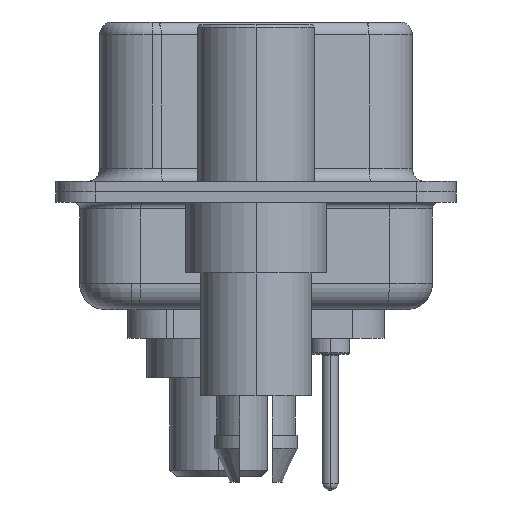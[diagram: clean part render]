
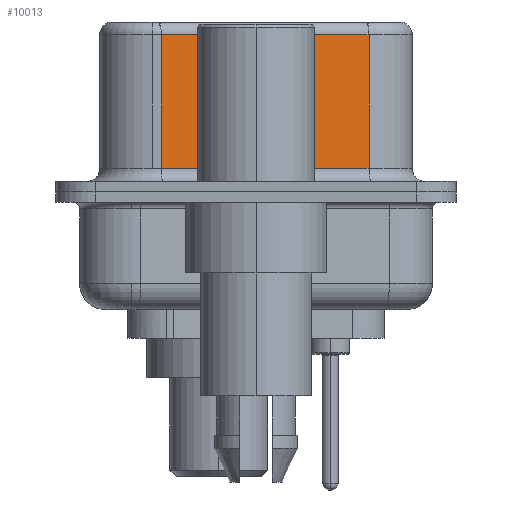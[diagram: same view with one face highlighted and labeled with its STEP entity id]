
A CAD part, left-side view. The second image highlights one B-rep face of the part: STEP entity #10013.
In plain terms, the highlighted planar face has unit normal (-0.985, -0.174, 0).
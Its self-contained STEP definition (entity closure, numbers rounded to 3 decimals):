
#69 = DIRECTION ( 'NONE',  ( 0.174, -0.985, 0. ) ) ;
#241 = VERTEX_POINT ( 'NONE', #258 ) ;
#258 = CARTESIAN_POINT ( 'NONE',  ( 3.73, 3.628, 0.9 ) ) ;
#412 = VERTEX_POINT ( 'NONE', #14796 ) ;
#1523 = VECTOR ( 'NONE', #13945, 1000. ) ;
#3657 = AXIS2_PLACEMENT_3D ( 'NONE', #19100, #8896, #8847 ) ;
#3812 = EDGE_CURVE ( 'NONE', #241, #412, #6726, .T. ) ;
#3997 = CARTESIAN_POINT ( 'NONE',  ( 3.73, 3.628, 6.52 ) ) ;
#5882 = ORIENTED_EDGE ( 'NONE', *, *, #21148, .T. ) ;
#6597 = VECTOR ( 'NONE', #19282, 1000. ) ;
#6726 = LINE ( 'NONE', #16814, #10634 ) ;
#8847 = DIRECTION ( 'NONE',  ( -0.174, 0.985, 0. ) ) ;
#8885 = EDGE_LOOP ( 'NONE', ( #20170, #19002, #5882, #21548 ) ) ;
#8896 = DIRECTION ( 'NONE',  ( 0.985, 0.174, 0. ) ) ;
#9167 = EDGE_CURVE ( 'NONE', #15910, #17161, #15515, .T. ) ;
#9474 = FACE_OUTER_BOUND ( 'NONE', #8885, .T. ) ;
#10013 = ADVANCED_FACE ( 'NONE', ( #9474 ), #15178, .F. ) ;
#10414 = LINE ( 'NONE', #3997, #1523 ) ;
#10546 = CARTESIAN_POINT ( 'NONE',  ( 5.132, -4.322, 6.52 ) ) ;
#10614 = DIRECTION ( 'NONE',  ( 0., 0., -1. ) ) ;
#10634 = VECTOR ( 'NONE', #69, 1000. ) ;
#11352 = LINE ( 'NONE', #10546, #19571 ) ;
#13945 = DIRECTION ( 'NONE',  ( 0., 0., -1. ) ) ;
#14779 = CARTESIAN_POINT ( 'NONE',  ( 3.73, 3.628, 6.02 ) ) ;
#14796 = CARTESIAN_POINT ( 'NONE',  ( 5.132, -4.322, 0.9 ) ) ;
#15178 = PLANE ( 'NONE',  #3657 ) ;
#15515 = LINE ( 'NONE', #16932, #6597 ) ;
#15910 = VERTEX_POINT ( 'NONE', #18822 ) ;
#16814 = CARTESIAN_POINT ( 'NONE',  ( 5.132, -4.322, 0.9 ) ) ;
#16932 = CARTESIAN_POINT ( 'NONE',  ( 5.132, -4.322, 6.02 ) ) ;
#17161 = VERTEX_POINT ( 'NONE', #14779 ) ;
#17542 = EDGE_CURVE ( 'NONE', #15910, #412, #11352, .T. ) ;
#18822 = CARTESIAN_POINT ( 'NONE',  ( 5.132, -4.322, 6.02 ) ) ;
#19002 = ORIENTED_EDGE ( 'NONE', *, *, #9167, .T. ) ;
#19100 = CARTESIAN_POINT ( 'NONE',  ( 5.132, -4.322, 6.52 ) ) ;
#19282 = DIRECTION ( 'NONE',  ( -0.174, 0.985, 0. ) ) ;
#19571 = VECTOR ( 'NONE', #10614, 1000. ) ;
#20170 = ORIENTED_EDGE ( 'NONE', *, *, #17542, .F. ) ;
#21148 = EDGE_CURVE ( 'NONE', #17161, #241, #10414, .T. ) ;
#21548 = ORIENTED_EDGE ( 'NONE', *, *, #3812, .T. ) ;
